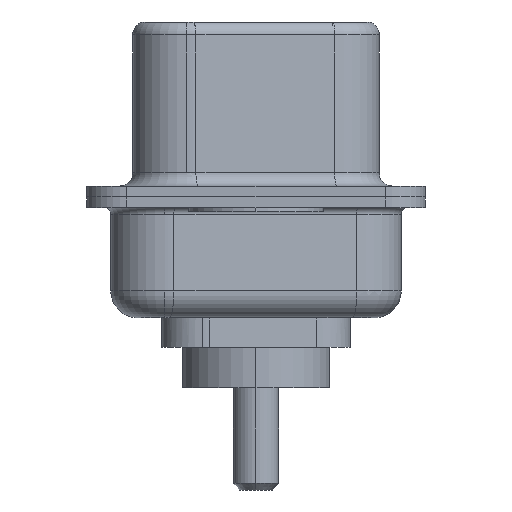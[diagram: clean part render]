
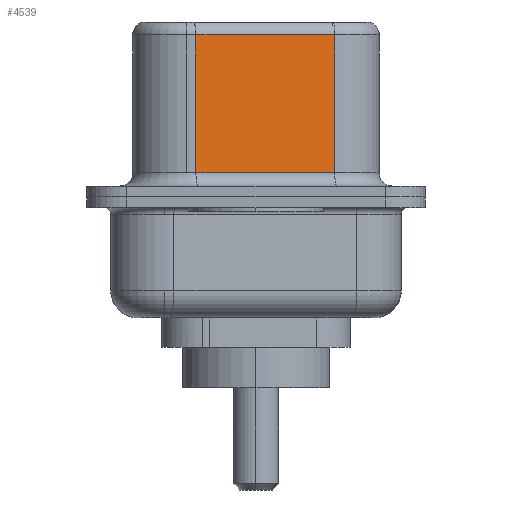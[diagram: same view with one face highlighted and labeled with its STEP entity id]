
A CAD part, left-side view. The second image highlights one B-rep face of the part: STEP entity #4539.
In plain terms, the highlighted planar face has unit normal (-0.985, -0.174, 0).
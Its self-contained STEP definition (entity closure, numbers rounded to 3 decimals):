
#105 = DIRECTION ( 'NONE',  ( -0.174, 0.985, 0. ) ) ;
#162 = VERTEX_POINT ( 'NONE', #8922 ) ;
#280 = DIRECTION ( 'NONE',  ( 0.985, 0.174, 0. ) ) ;
#1255 = VECTOR ( 'NONE', #2434, 1000. ) ;
#1491 = VECTOR ( 'NONE', #105, 1000. ) ;
#1617 = VERTEX_POINT ( 'NONE', #12973 ) ;
#2434 = DIRECTION ( 'NONE',  ( 0., 0., -1. ) ) ;
#2488 = DIRECTION ( 'NONE',  ( -0.174, 0.985, 0. ) ) ;
#3000 = EDGE_LOOP ( 'NONE', ( #5522, #7662, #10185, #11490 ) ) ;
#4539 = ADVANCED_FACE ( 'NONE', ( #5190 ), #13399, .F. ) ;
#5190 = FACE_OUTER_BOUND ( 'NONE', #3000, .T. ) ;
#5522 = ORIENTED_EDGE ( 'NONE', *, *, #14007, .F. ) ;
#5927 = EDGE_CURVE ( 'NONE', #1617, #162, #9922, .T. ) ;
#6033 = VECTOR ( 'NONE', #10967, 1000. ) ;
#6068 = CARTESIAN_POINT ( 'NONE',  ( 4.58, -2.927, 0.9 ) ) ;
#6347 = DIRECTION ( 'NONE',  ( 0.174, -0.985, 0. ) ) ;
#6512 = VERTEX_POINT ( 'NONE', #10718 ) ;
#7662 = ORIENTED_EDGE ( 'NONE', *, *, #9500, .T. ) ;
#7675 = CARTESIAN_POINT ( 'NONE',  ( 4.58, -2.927, 6.52 ) ) ;
#7798 = CARTESIAN_POINT ( 'NONE',  ( 4.58, -2.927, 6.02 ) ) ;
#8011 = CARTESIAN_POINT ( 'NONE',  ( 4.58, -2.927, 6.52 ) ) ;
#8612 = EDGE_CURVE ( 'NONE', #162, #6512, #12453, .T. ) ;
#8816 = AXIS2_PLACEMENT_3D ( 'NONE', #8011, #280, #2488 ) ;
#8922 = CARTESIAN_POINT ( 'NONE',  ( 3.67, 2.233, 0.9 ) ) ;
#9500 = EDGE_CURVE ( 'NONE', #13029, #1617, #12259, .T. ) ;
#9507 = VECTOR ( 'NONE', #6347, 1000. ) ;
#9601 = LINE ( 'NONE', #7675, #6033 ) ;
#9922 = LINE ( 'NONE', #13495, #1255 ) ;
#10185 = ORIENTED_EDGE ( 'NONE', *, *, #5927, .T. ) ;
#10718 = CARTESIAN_POINT ( 'NONE',  ( 4.58, -2.927, 0.9 ) ) ;
#10967 = DIRECTION ( 'NONE',  ( 0., 0., -1. ) ) ;
#11490 = ORIENTED_EDGE ( 'NONE', *, *, #8612, .T. ) ;
#12259 = LINE ( 'NONE', #7798, #1491 ) ;
#12453 = LINE ( 'NONE', #6068, #9507 ) ;
#12572 = CARTESIAN_POINT ( 'NONE',  ( 4.58, -2.927, 6.02 ) ) ;
#12973 = CARTESIAN_POINT ( 'NONE',  ( 3.67, 2.233, 6.02 ) ) ;
#13029 = VERTEX_POINT ( 'NONE', #12572 ) ;
#13399 = PLANE ( 'NONE',  #8816 ) ;
#13495 = CARTESIAN_POINT ( 'NONE',  ( 3.67, 2.233, 6.52 ) ) ;
#14007 = EDGE_CURVE ( 'NONE', #13029, #6512, #9601, .T. ) ;
